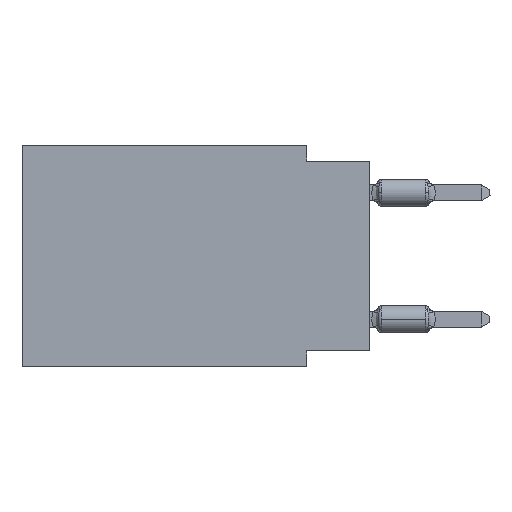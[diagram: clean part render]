
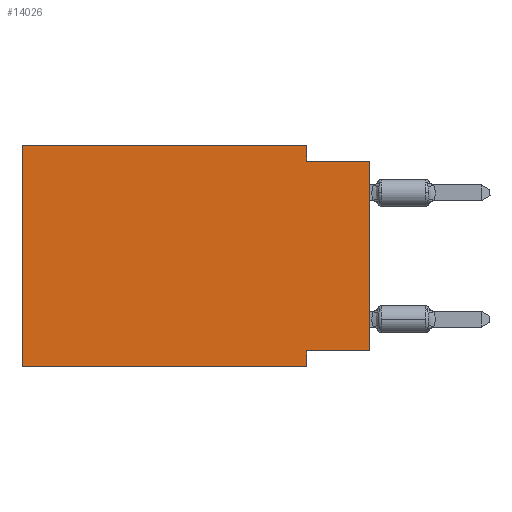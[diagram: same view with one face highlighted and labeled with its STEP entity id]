
A CAD part, left-side view. The second image highlights one B-rep face of the part: STEP entity #14026.
In plain terms, the highlighted planar face has unit normal (-1, 0, 0).
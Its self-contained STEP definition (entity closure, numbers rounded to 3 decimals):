
#2054 = LINE ( 'NONE', #20194, #37875 ) ;
#2729 = VERTEX_POINT ( 'NONE', #17612 ) ;
#3468 = CARTESIAN_POINT ( 'NONE',  ( 0., 2.54, -8.89 ) ) ;
#3589 = CARTESIAN_POINT ( 'NONE',  ( 0., 2.54, 0. ) ) ;
#3874 = VECTOR ( 'NONE', #7043, 1000. ) ;
#5432 = VECTOR ( 'NONE', #24142, 1000. ) ;
#5963 = DIRECTION ( 'NONE',  ( 0., 0., -1. ) ) ;
#6292 = ORIENTED_EDGE ( 'NONE', *, *, #10524, .F. ) ;
#7043 = DIRECTION ( 'NONE',  ( 0., 0., 1. ) ) ;
#7399 = VERTEX_POINT ( 'NONE', #3468 ) ;
#7934 = LINE ( 'NONE', #28805, #33950 ) ;
#8716 = FACE_OUTER_BOUND ( 'NONE', #10668, .T. ) ;
#9209 = VECTOR ( 'NONE', #15494, 1000. ) ;
#10524 = EDGE_CURVE ( 'NONE', #2729, #24212, #21726, .T. ) ;
#10644 = CARTESIAN_POINT ( 'NONE',  ( 0., 13.97, 0. ) ) ;
#10668 = EDGE_LOOP ( 'NONE', ( #12359, #17392, #6292, #15736, #11327, #22020, #31901, #19181 ) ) ;
#11327 = ORIENTED_EDGE ( 'NONE', *, *, #30213, .F. ) ;
#11601 = DIRECTION ( 'NONE',  ( 0., 1., 0. ) ) ;
#12359 = ORIENTED_EDGE ( 'NONE', *, *, #33596, .T. ) ;
#12949 = VERTEX_POINT ( 'NONE', #25261 ) ;
#14026 = ADVANCED_FACE ( 'NONE', ( #8716 ), #29569, .F. ) ;
#14319 = VERTEX_POINT ( 'NONE', #29345 ) ;
#14364 = DIRECTION ( 'NONE',  ( 0., -1., 0. ) ) ;
#15494 = DIRECTION ( 'NONE',  ( 0., 0., -1. ) ) ;
#15736 = ORIENTED_EDGE ( 'NONE', *, *, #19360, .F. ) ;
#16970 = AXIS2_PLACEMENT_3D ( 'NONE', #35595, #20797, #5963 ) ;
#17392 = ORIENTED_EDGE ( 'NONE', *, *, #26021, .F. ) ;
#17612 = CARTESIAN_POINT ( 'NONE',  ( 0., 2.54, 0. ) ) ;
#18343 = VECTOR ( 'NONE', #26196, 1000. ) ;
#18875 = CARTESIAN_POINT ( 'NONE',  ( 0., 0., -0.635 ) ) ;
#18942 = LINE ( 'NONE', #27914, #3874 ) ;
#19181 = ORIENTED_EDGE ( 'NONE', *, *, #36411, .F. ) ;
#19360 = EDGE_CURVE ( 'NONE', #34984, #2729, #38033, .T. ) ;
#20194 = CARTESIAN_POINT ( 'NONE',  ( 0., 0., -8.255 ) ) ;
#20311 = DIRECTION ( 'NONE',  ( 0., -1., 0. ) ) ;
#20331 = CARTESIAN_POINT ( 'NONE',  ( 0., 0., -0.635 ) ) ;
#20571 = CARTESIAN_POINT ( 'NONE',  ( 0., 2.54, -8.89 ) ) ;
#20797 = DIRECTION ( 'NONE',  ( 1., 0., 0. ) ) ;
#21726 = LINE ( 'NONE', #3589, #9209 ) ;
#22020 = ORIENTED_EDGE ( 'NONE', *, *, #32111, .T. ) ;
#23698 = VERTEX_POINT ( 'NONE', #18875 ) ;
#24142 = DIRECTION ( 'NONE',  ( 0., 0., 1. ) ) ;
#24212 = VERTEX_POINT ( 'NONE', #31494 ) ;
#25261 = CARTESIAN_POINT ( 'NONE',  ( 0., 2.54, -8.255 ) ) ;
#26021 = EDGE_CURVE ( 'NONE', #24212, #23698, #29108, .T. ) ;
#26196 = DIRECTION ( 'NONE',  ( 0., -1., 0. ) ) ;
#26632 = VECTOR ( 'NONE', #37514, 1000. ) ;
#27859 = CARTESIAN_POINT ( 'NONE',  ( 0., 13.97, -8.89 ) ) ;
#27914 = CARTESIAN_POINT ( 'NONE',  ( 0., 13.97, 0. ) ) ;
#28805 = CARTESIAN_POINT ( 'NONE',  ( 0., 13.97, -8.89 ) ) ;
#29108 = LINE ( 'NONE', #20331, #18343 ) ;
#29345 = CARTESIAN_POINT ( 'NONE',  ( 0., 0., -8.255 ) ) ;
#29373 = VERTEX_POINT ( 'NONE', #27859 ) ;
#29569 = PLANE ( 'NONE',  #16970 ) ;
#29992 = LINE ( 'NONE', #38175, #5432 ) ;
#30213 = EDGE_CURVE ( 'NONE', #29373, #34984, #18942, .T. ) ;
#31005 = VECTOR ( 'NONE', #20311, 1000. ) ;
#31494 = CARTESIAN_POINT ( 'NONE',  ( 0., 2.54, -0.635 ) ) ;
#31901 = ORIENTED_EDGE ( 'NONE', *, *, #33770, .F. ) ;
#32111 = EDGE_CURVE ( 'NONE', #29373, #7399, #7934, .T. ) ;
#32197 = CARTESIAN_POINT ( 'NONE',  ( 0., 13.97, 0. ) ) ;
#33596 = EDGE_CURVE ( 'NONE', #14319, #23698, #29992, .T. ) ;
#33770 = EDGE_CURVE ( 'NONE', #12949, #7399, #34595, .T. ) ;
#33950 = VECTOR ( 'NONE', #14364, 1000. ) ;
#34595 = LINE ( 'NONE', #20571, #26632 ) ;
#34984 = VERTEX_POINT ( 'NONE', #10644 ) ;
#35595 = CARTESIAN_POINT ( 'NONE',  ( 0., 13.97, 0. ) ) ;
#36411 = EDGE_CURVE ( 'NONE', #14319, #12949, #2054, .T. ) ;
#37514 = DIRECTION ( 'NONE',  ( 0., 0., -1. ) ) ;
#37875 = VECTOR ( 'NONE', #11601, 1000. ) ;
#38033 = LINE ( 'NONE', #32197, #31005 ) ;
#38175 = CARTESIAN_POINT ( 'NONE',  ( 0., 0., 0. ) ) ;
